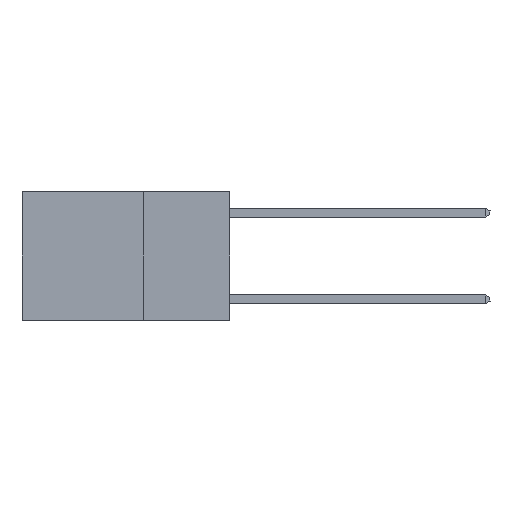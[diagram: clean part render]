
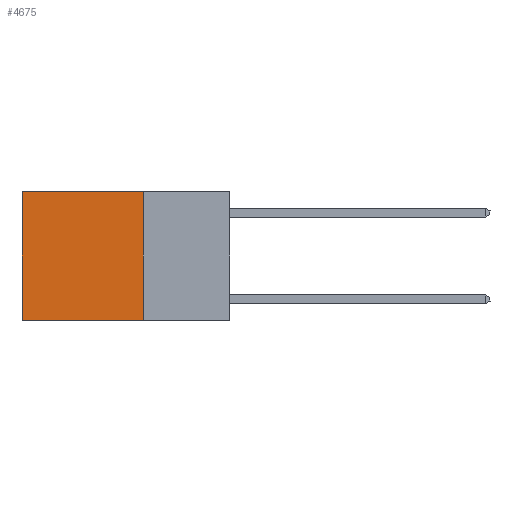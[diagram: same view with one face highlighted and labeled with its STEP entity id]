
A CAD part, left-side view. The second image highlights one B-rep face of the part: STEP entity #4675.
In plain terms, the highlighted planar face has unit normal (-1, 0, 0).
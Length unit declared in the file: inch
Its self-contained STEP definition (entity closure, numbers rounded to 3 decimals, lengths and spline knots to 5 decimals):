
#510 = CARTESIAN_POINT ( 'NONE',  ( 0.2625, 0.25, -0.37 ) ) ;
#806 = DIRECTION ( 'NONE',  ( 0., 0., -1. ) ) ;
#884 = EDGE_CURVE ( 'NONE', #1078, #4654, #7126, .T. ) ;
#1078 = VERTEX_POINT ( 'NONE', #510 ) ;
#1477 = CARTESIAN_POINT ( 'NONE',  ( 0.2625, 0.6, 0. ) ) ;
#1503 = VERTEX_POINT ( 'NONE', #1477 ) ;
#1795 = LINE ( 'NONE', #9756, #2021 ) ;
#2021 = VECTOR ( 'NONE', #5669, 39.37008 ) ;
#2279 = ORIENTED_EDGE ( 'NONE', *, *, #9806, .T. ) ;
#2482 = DIRECTION ( 'NONE',  ( 0., 1., 0. ) ) ;
#2548 = LINE ( 'NONE', #7570, #11497 ) ;
#2701 = ORIENTED_EDGE ( 'NONE', *, *, #5485, .F. ) ;
#2836 = VECTOR ( 'NONE', #6339, 39.37008 ) ;
#3083 = AXIS2_PLACEMENT_3D ( 'NONE', #4484, #10351, #12402 ) ;
#3369 = FACE_OUTER_BOUND ( 'NONE', #9165, .T. ) ;
#3675 = VERTEX_POINT ( 'NONE', #4014 ) ;
#4014 = CARTESIAN_POINT ( 'NONE',  ( 0.2625, 0.25, 0. ) ) ;
#4484 = CARTESIAN_POINT ( 'NONE',  ( 0.2625, 0.25, 0. ) ) ;
#4654 = VERTEX_POINT ( 'NONE', #12216 ) ;
#4675 = ADVANCED_FACE ( 'NONE', ( #3369 ), #8319, .F. ) ;
#5485 = EDGE_CURVE ( 'NONE', #3675, #1078, #1795, .T. ) ;
#5669 = DIRECTION ( 'NONE',  ( 0., 0., -1. ) ) ;
#6146 = CARTESIAN_POINT ( 'NONE',  ( 0.2625, 0.25, -0.37 ) ) ;
#6339 = DIRECTION ( 'NONE',  ( 0., 1., 0. ) ) ;
#7126 = LINE ( 'NONE', #6146, #2836 ) ;
#7570 = CARTESIAN_POINT ( 'NONE',  ( 0.2625, 0.25, 0. ) ) ;
#7735 = CARTESIAN_POINT ( 'NONE',  ( 0.2625, 0.6, 0. ) ) ;
#8319 = PLANE ( 'NONE',  #3083 ) ;
#8593 = ORIENTED_EDGE ( 'NONE', *, *, #10648, .T. ) ;
#8762 = LINE ( 'NONE', #7735, #11879 ) ;
#9165 = EDGE_LOOP ( 'NONE', ( #2279, #12446, #2701, #8593 ) ) ;
#9756 = CARTESIAN_POINT ( 'NONE',  ( 0.2625, 0.25, 0. ) ) ;
#9806 = EDGE_CURVE ( 'NONE', #1503, #4654, #8762, .T. ) ;
#10351 = DIRECTION ( 'NONE',  ( 1., 0., 0. ) ) ;
#10648 = EDGE_CURVE ( 'NONE', #3675, #1503, #2548, .T. ) ;
#11497 = VECTOR ( 'NONE', #2482, 39.37008 ) ;
#11879 = VECTOR ( 'NONE', #806, 39.37008 ) ;
#12216 = CARTESIAN_POINT ( 'NONE',  ( 0.2625, 0.6, -0.37 ) ) ;
#12402 = DIRECTION ( 'NONE',  ( 0., 0., -1. ) ) ;
#12446 = ORIENTED_EDGE ( 'NONE', *, *, #884, .F. ) ;
